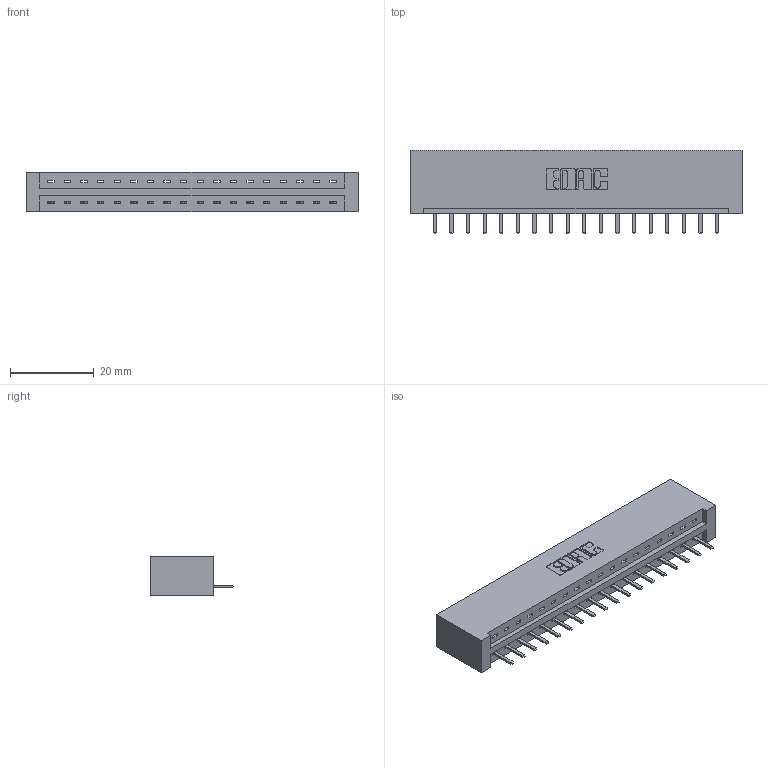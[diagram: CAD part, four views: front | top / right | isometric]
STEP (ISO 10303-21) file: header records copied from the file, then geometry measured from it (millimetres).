
FILE_DESCRIPTION (( 'STEP AP203' ), '1' );
FILE_NAME ('387-018-520-101.STEP', '2019-10-02T19:46:22', ( '' ), ( '' ), 'SwSTEP 2.0', 'SolidWorks 2016', '' );
FILE_SCHEMA (( 'CONFIG_CONTROL_DESIGN' ));
Length unit declared in the file: inch
Products named in the file (3): 337 Part_No Mounting Lugs; 345-292-001_345-293-120; 387-018-520-101
Assembly tree (19 placements, depth 2):
  387-018-520-101
    337 Part_No Mounting Lugs
    345-292-001_345-293-120  x18
Bounding box: 79.2 x 20.02 x 9.4 mm (x, y, z)
Volume: 8617.8 mm3; surface area: 8567.1 mm2
Topology: 19 solids, 19 shells, 1294 faces, 3815 edges, 2494 vertices
Faces by surface type: plane 930, cylinder 364
Entity records: 16321 total; most frequent: CARTESIAN_POINT 2860, ORIENTED_EDGE 2802, DIRECTION 2437, EDGE_CURVE 1401, VECTOR 1277, LINE 1277, VERTEX_POINT 930, AXIS2_PLACEMENT_3D 580
